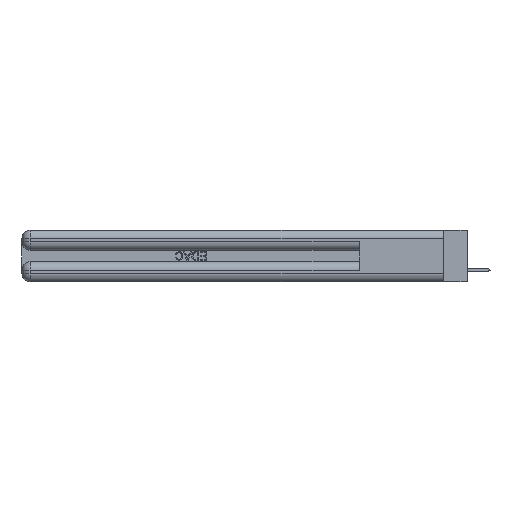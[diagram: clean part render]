
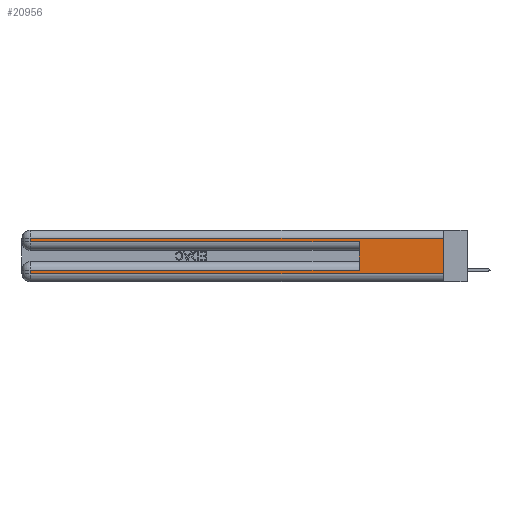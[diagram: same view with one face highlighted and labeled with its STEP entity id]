
A CAD part, left-side view. The second image highlights one B-rep face of the part: STEP entity #20956.
In plain terms, the highlighted planar face has unit normal (-1, 0, 0).
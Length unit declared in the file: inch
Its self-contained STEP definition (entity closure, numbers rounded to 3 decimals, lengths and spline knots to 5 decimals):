
#1 = LINE ( 'NONE', #26418, #33416 ) ;
#1058 = ORIENTED_EDGE ( 'NONE', *, *, #7906, .T. ) ;
#1363 = CARTESIAN_POINT ( 'NONE',  ( 0., 2.94, 0.31 ) ) ;
#2032 = DIRECTION ( 'NONE',  ( 0., 0., -1. ) ) ;
#2276 = CARTESIAN_POINT ( 'NONE',  ( 0., 0., 0.37 ) ) ;
#2565 = ORIENTED_EDGE ( 'NONE', *, *, #49636, .T. ) ;
#2860 = VECTOR ( 'NONE', #2032, 39.37008 ) ;
#3311 = VERTEX_POINT ( 'NONE', #22295 ) ;
#4053 = VERTEX_POINT ( 'NONE', #35062 ) ;
#5653 = EDGE_LOOP ( 'NONE', ( #33007, #50087, #6100, #22853, #25502, #31967, #2565, #1058 ) ) ;
#6021 = VECTOR ( 'NONE', #19660, 39.37008 ) ;
#6100 = ORIENTED_EDGE ( 'NONE', *, *, #48560, .T. ) ;
#7856 = CARTESIAN_POINT ( 'NONE',  ( 0., 2.94, 0.06 ) ) ;
#7906 = EDGE_CURVE ( 'NONE', #46860, #48966, #37604, .T. ) ;
#7948 = DIRECTION ( 'NONE',  ( 0., 1., 0. ) ) ;
#9895 = DIRECTION ( 'NONE',  ( 0., 0., 1. ) ) ;
#10227 = PLANE ( 'NONE',  #50191 ) ;
#10268 = CARTESIAN_POINT ( 'NONE',  ( 0., 0., 0.06 ) ) ;
#10780 = LINE ( 'NONE', #34199, #22779 ) ;
#12425 = EDGE_CURVE ( 'NONE', #42651, #48966, #35115, .T. ) ;
#12901 = CARTESIAN_POINT ( 'NONE',  ( 0., 0., 0.06 ) ) ;
#14147 = CARTESIAN_POINT ( 'NONE',  ( 0., 0., 0.31 ) ) ;
#15383 = EDGE_CURVE ( 'NONE', #25261, #3311, #10780, .T. ) ;
#16753 = LINE ( 'NONE', #39776, #6021 ) ;
#18814 = LINE ( 'NONE', #28300, #20677 ) ;
#19660 = DIRECTION ( 'NONE',  ( 0., 0., -1. ) ) ;
#20677 = VECTOR ( 'NONE', #7948, 39.37008 ) ;
#20956 = ADVANCED_FACE ( 'NONE', ( #24753 ), #10227, .F. ) ;
#22295 = CARTESIAN_POINT ( 'NONE',  ( 0., 0.6, 0.285 ) ) ;
#22779 = VECTOR ( 'NONE', #49967, 39.37008 ) ;
#22853 = ORIENTED_EDGE ( 'NONE', *, *, #15383, .T. ) ;
#24753 = FACE_OUTER_BOUND ( 'NONE', #5653, .T. ) ;
#25261 = VERTEX_POINT ( 'NONE', #25645 ) ;
#25502 = ORIENTED_EDGE ( 'NONE', *, *, #47241, .F. ) ;
#25645 = CARTESIAN_POINT ( 'NONE',  ( 0., 2.94, 0.285 ) ) ;
#26130 = VECTOR ( 'NONE', #51409, 39.37008 ) ;
#26418 = CARTESIAN_POINT ( 'NONE',  ( 0., 0., 0.085 ) ) ;
#28300 = CARTESIAN_POINT ( 'NONE',  ( 0., 0., 0.31 ) ) ;
#30142 = DIRECTION ( 'NONE',  ( 0., 1., 0. ) ) ;
#30202 = DIRECTION ( 'NONE',  ( 1., 0., 0. ) ) ;
#30451 = EDGE_CURVE ( 'NONE', #42651, #46398, #18814, .T. ) ;
#31908 = VECTOR ( 'NONE', #9895, 39.37008 ) ;
#31967 = ORIENTED_EDGE ( 'NONE', *, *, #36838, .T. ) ;
#32799 = LINE ( 'NONE', #51288, #39847 ) ;
#33007 = ORIENTED_EDGE ( 'NONE', *, *, #12425, .F. ) ;
#33416 = VECTOR ( 'NONE', #30142, 39.37008 ) ;
#34199 = CARTESIAN_POINT ( 'NONE',  ( 0., 0., 0.285 ) ) ;
#34647 = DIRECTION ( 'NONE',  ( 0., 0., -1. ) ) ;
#35062 = CARTESIAN_POINT ( 'NONE',  ( 0., 0.6, 0.085 ) ) ;
#35115 = LINE ( 'NONE', #50564, #2860 ) ;
#36387 = LINE ( 'NONE', #38622, #31908 ) ;
#36838 = EDGE_CURVE ( 'NONE', #4053, #40285, #1, .T. ) ;
#37604 = LINE ( 'NONE', #10268, #26130 ) ;
#38622 = CARTESIAN_POINT ( 'NONE',  ( 0., 0.6, 0.145 ) ) ;
#39776 = CARTESIAN_POINT ( 'NONE',  ( 0., 2.94, 0.37 ) ) ;
#39847 = VECTOR ( 'NONE', #47604, 39.37008 ) ;
#40285 = VERTEX_POINT ( 'NONE', #50532 ) ;
#42651 = VERTEX_POINT ( 'NONE', #14147 ) ;
#46398 = VERTEX_POINT ( 'NONE', #1363 ) ;
#46860 = VERTEX_POINT ( 'NONE', #7856 ) ;
#47241 = EDGE_CURVE ( 'NONE', #4053, #3311, #36387, .T. ) ;
#47604 = DIRECTION ( 'NONE',  ( 0., 0., -1. ) ) ;
#48560 = EDGE_CURVE ( 'NONE', #46398, #25261, #32799, .T. ) ;
#48966 = VERTEX_POINT ( 'NONE', #12901 ) ;
#49636 = EDGE_CURVE ( 'NONE', #40285, #46860, #16753, .T. ) ;
#49967 = DIRECTION ( 'NONE',  ( 0., -1., 0. ) ) ;
#50087 = ORIENTED_EDGE ( 'NONE', *, *, #30451, .T. ) ;
#50191 = AXIS2_PLACEMENT_3D ( 'NONE', #2276, #30202, #34647 ) ;
#50532 = CARTESIAN_POINT ( 'NONE',  ( 0., 2.94, 0.085 ) ) ;
#50564 = CARTESIAN_POINT ( 'NONE',  ( 0., 0., 0.37 ) ) ;
#51288 = CARTESIAN_POINT ( 'NONE',  ( 0., 2.94, 0.37 ) ) ;
#51409 = DIRECTION ( 'NONE',  ( 0., -1., 0. ) ) ;
